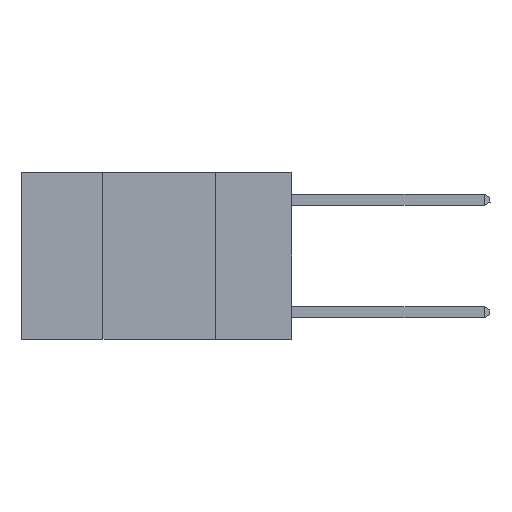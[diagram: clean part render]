
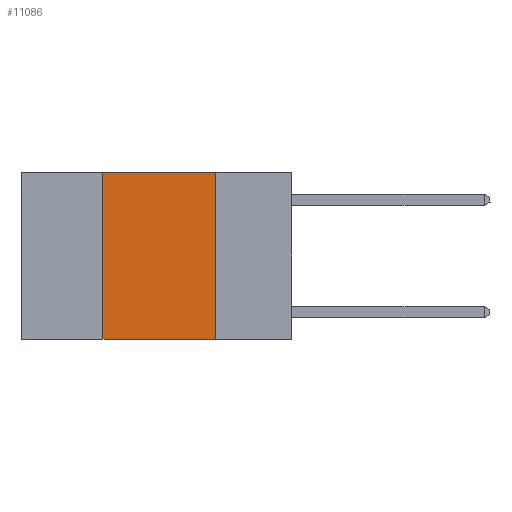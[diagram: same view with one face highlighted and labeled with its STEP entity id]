
A CAD part, left-side view. The second image highlights one B-rep face of the part: STEP entity #11086.
In plain terms, the highlighted planar face has unit normal (-1, 0, 0).
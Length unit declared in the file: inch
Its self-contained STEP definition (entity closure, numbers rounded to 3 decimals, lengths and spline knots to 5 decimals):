
#627 = CARTESIAN_POINT ( 'NONE',  ( 0., 0.42, 0. ) ) ;
#1069 = EDGE_CURVE ( 'NONE', #9827, #1748, #5161, .T. ) ;
#1748 = VERTEX_POINT ( 'NONE', #627 ) ;
#2299 = VERTEX_POINT ( 'NONE', #9246 ) ;
#2384 = CARTESIAN_POINT ( 'NONE',  ( 0., 0.17, 0. ) ) ;
#2924 = EDGE_CURVE ( 'NONE', #2299, #8669, #10597, .T. ) ;
#2954 = CARTESIAN_POINT ( 'NONE',  ( 0., 0.6, -0.37 ) ) ;
#3930 = DIRECTION ( 'NONE',  ( 0., -1., 0. ) ) ;
#4546 = AXIS2_PLACEMENT_3D ( 'NONE', #10137, #11837, #6490 ) ;
#4715 = CARTESIAN_POINT ( 'NONE',  ( 0., 0.17, -0.37 ) ) ;
#5161 = LINE ( 'NONE', #10752, #9819 ) ;
#5682 = LINE ( 'NONE', #2954, #10294 ) ;
#6327 = ORIENTED_EDGE ( 'NONE', *, *, #8755, .T. ) ;
#6490 = DIRECTION ( 'NONE',  ( 0., 0., -1. ) ) ;
#7267 = CARTESIAN_POINT ( 'NONE',  ( 0., 0.6, 0. ) ) ;
#7492 = DIRECTION ( 'NONE',  ( 0., 0., 1. ) ) ;
#7604 = EDGE_LOOP ( 'NONE', ( #11479, #9669, #8371, #6327 ) ) ;
#7869 = VECTOR ( 'NONE', #8248, 39.37008 ) ;
#8248 = DIRECTION ( 'NONE',  ( 0., -1., 0. ) ) ;
#8371 = ORIENTED_EDGE ( 'NONE', *, *, #1069, .F. ) ;
#8669 = VERTEX_POINT ( 'NONE', #4715 ) ;
#8755 = EDGE_CURVE ( 'NONE', #9827, #8669, #5682, .T. ) ;
#9246 = CARTESIAN_POINT ( 'NONE',  ( 0., 0.17, 0. ) ) ;
#9669 = ORIENTED_EDGE ( 'NONE', *, *, #9991, .F. ) ;
#9819 = VECTOR ( 'NONE', #7492, 39.37008 ) ;
#9827 = VERTEX_POINT ( 'NONE', #9831 ) ;
#9831 = CARTESIAN_POINT ( 'NONE',  ( 0., 0.42, -0.37 ) ) ;
#9991 = EDGE_CURVE ( 'NONE', #1748, #2299, #10145, .T. ) ;
#10137 = CARTESIAN_POINT ( 'NONE',  ( 0., 0.6, 0. ) ) ;
#10145 = LINE ( 'NONE', #7267, #7869 ) ;
#10294 = VECTOR ( 'NONE', #3930, 39.37008 ) ;
#10315 = VECTOR ( 'NONE', #10411, 39.37008 ) ;
#10411 = DIRECTION ( 'NONE',  ( 0., 0., -1. ) ) ;
#10597 = LINE ( 'NONE', #2384, #10315 ) ;
#10663 = FACE_OUTER_BOUND ( 'NONE', #7604, .T. ) ;
#10752 = CARTESIAN_POINT ( 'NONE',  ( 0., 0.42, 0. ) ) ;
#10990 = PLANE ( 'NONE',  #4546 ) ;
#11086 = ADVANCED_FACE ( 'NONE', ( #10663 ), #10990, .F. ) ;
#11479 = ORIENTED_EDGE ( 'NONE', *, *, #2924, .F. ) ;
#11837 = DIRECTION ( 'NONE',  ( 1., 0., 0. ) ) ;
